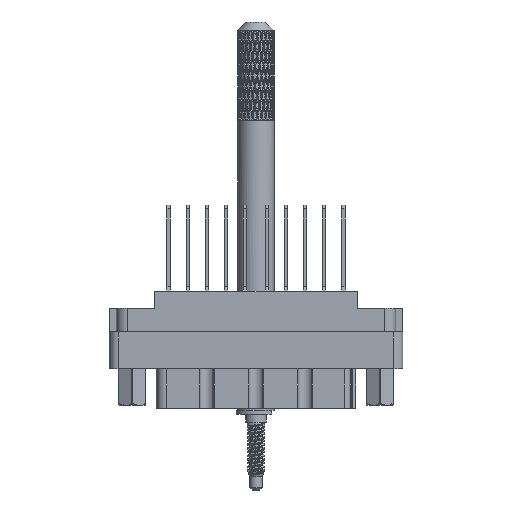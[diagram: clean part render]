
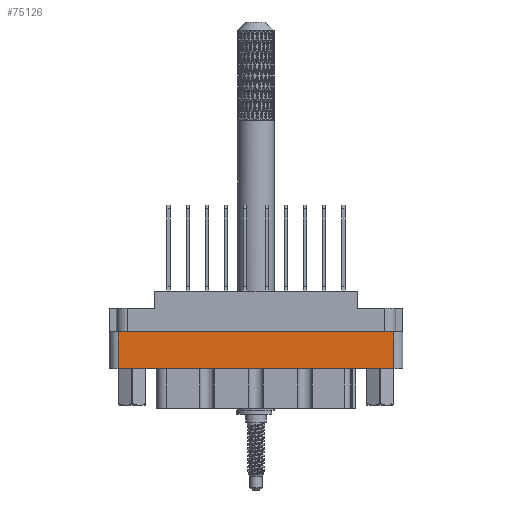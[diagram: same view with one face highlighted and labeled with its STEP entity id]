
A CAD part, front view. The second image highlights one B-rep face of the part: STEP entity #75126.
In plain terms, the highlighted planar face has unit normal (0, -1, 0).
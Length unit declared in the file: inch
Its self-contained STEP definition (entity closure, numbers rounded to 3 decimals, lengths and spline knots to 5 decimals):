
#4861 = AXIS2_PLACEMENT_3D ( 'NONE', #44640, #80924, #97009 ) ;
#24550 = EDGE_CURVE ( 'NONE', #48328, #51633, #29432, .T. ) ;
#24558 = CARTESIAN_POINT ( 'NONE',  ( 0.938, -0.438, -0.529 ) ) ;
#25477 = VECTOR ( 'NONE', #105603, 39.37008 ) ;
#27596 = LINE ( 'NONE', #65960, #101426 ) ;
#27687 = EDGE_CURVE ( 'NONE', #79325, #51633, #27596, .T. ) ;
#29432 = LINE ( 'NONE', #65595, #82760 ) ;
#34416 = DIRECTION ( 'NONE',  ( 0., 0., -1. ) ) ;
#35838 = PLANE ( 'NONE',  #4861 ) ;
#39765 = EDGE_LOOP ( 'NONE', ( #80396, #101079, #79414, #78290 ) ) ;
#44640 = CARTESIAN_POINT ( 'NONE',  ( -1., -0.438, -0.798 ) ) ;
#45967 = CARTESIAN_POINT ( 'NONE',  ( 0.938, -0.438, -0.277 ) ) ;
#48186 = VERTEX_POINT ( 'NONE', #57445 ) ;
#48328 = VERTEX_POINT ( 'NONE', #24558 ) ;
#49555 = FACE_OUTER_BOUND ( 'NONE', #39765, .T. ) ;
#51437 = LINE ( 'NONE', #87946, #25477 ) ;
#51633 = VERTEX_POINT ( 'NONE', #45967 ) ;
#55982 = DIRECTION ( 'NONE',  ( 0., 0., 1. ) ) ;
#57445 = CARTESIAN_POINT ( 'NONE',  ( -0.938, -0.438, -0.529 ) ) ;
#65595 = CARTESIAN_POINT ( 'NONE',  ( 0.938, -0.438, -0.798 ) ) ;
#65960 = CARTESIAN_POINT ( 'NONE',  ( 0., -0.438, -0.277 ) ) ;
#75126 = ADVANCED_FACE ( 'NONE', ( #49555 ), #35838, .T. ) ;
#75742 = LINE ( 'NONE', #86757, #108564 ) ;
#78290 = ORIENTED_EDGE ( 'NONE', *, *, #24550, .T. ) ;
#79325 = VERTEX_POINT ( 'NONE', #95729 ) ;
#79414 = ORIENTED_EDGE ( 'NONE', *, *, #99578, .F. ) ;
#80396 = ORIENTED_EDGE ( 'NONE', *, *, #27687, .F. ) ;
#80924 = DIRECTION ( 'NONE',  ( 0., -1., 0. ) ) ;
#82760 = VECTOR ( 'NONE', #55982, 39.37008 ) ;
#86757 = CARTESIAN_POINT ( 'NONE',  ( -0.938, -0.438, -0.798 ) ) ;
#87946 = CARTESIAN_POINT ( 'NONE',  ( 0., -0.438, -0.529 ) ) ;
#91660 = EDGE_CURVE ( 'NONE', #79325, #48186, #75742, .T. ) ;
#93042 = DIRECTION ( 'NONE',  ( 1., 0., 0. ) ) ;
#95729 = CARTESIAN_POINT ( 'NONE',  ( -0.938, -0.438, -0.277 ) ) ;
#97009 = DIRECTION ( 'NONE',  ( 0., 0., -1. ) ) ;
#99578 = EDGE_CURVE ( 'NONE', #48328, #48186, #51437, .T. ) ;
#101079 = ORIENTED_EDGE ( 'NONE', *, *, #91660, .T. ) ;
#101426 = VECTOR ( 'NONE', #93042, 39.37008 ) ;
#105603 = DIRECTION ( 'NONE',  ( -1., 0., 0. ) ) ;
#108564 = VECTOR ( 'NONE', #34416, 39.37008 ) ;
